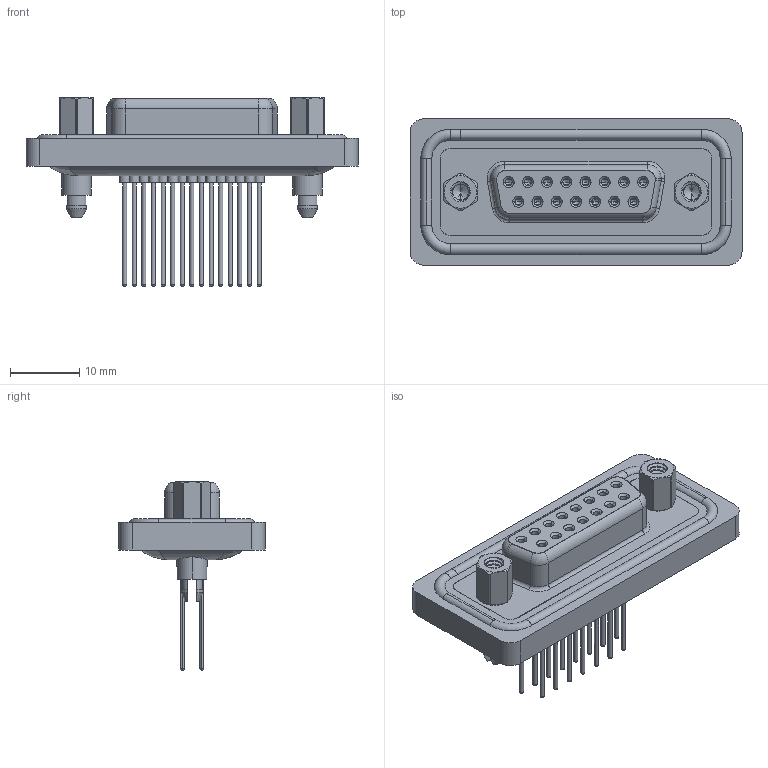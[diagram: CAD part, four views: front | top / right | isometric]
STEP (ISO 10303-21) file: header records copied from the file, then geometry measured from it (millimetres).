
FILE_DESCRIPTION (( 'STEP AP203' ), '1' );
FILE_NAME ('628-W15-321-013.STEP', '2020-09-11T23:25:36', ( '' ), ( '' ), 'SwSTEP 2.0', 'SolidWorks 2020', '' );
FILE_SCHEMA (( 'CONFIG_CONTROL_DESIGN' ));
Length unit declared in the file: millimetre
Products named in the file (8): 628W Housing_15 Contacts; 628W Waterproof Housing_15 Contacts BL; 628W Contact Row 1_21; 628W 4-40 Threaded Boardlock; 628W 4-40 Hex Standoff; 628-W15-321-013; 628W Contact Row 2_21; 628W Shell Front_15 Contacts
Assembly tree (22 placements, depth 2):
  628-W15-321-013
    628W Housing_15 Contacts
    628W Shell Front_15 Contacts
    628W Contact Row 1_21  x8
    628W Contact Row 2_21  x7
    628W 4-40 Threaded Boardlock  x2
    628W Waterproof Housing_15 Contacts BL
    628W 4-40 Hex Standoff  x2
Bounding box: 47.89 x 21.1 x 27.2 mm (x, y, z)
Volume: 5651.1 mm3; surface area: 9963.2 mm2
Topology: 23 solids, 23 shells, 1324 faces, 3196 edges, 1989 vertices
Faces by surface type: cylinder 563, plane 340, torus 260, cone 139, bspline 22
Entity records: 25350 total; most frequent: CARTESIAN_POINT 8378, DIRECTION 3481, ORIENTED_EDGE 3178, EDGE_CURVE 1589, AXIS2_PLACEMENT_3D 1441, VERTEX_POINT 1014, EDGE_LOOP 795, CIRCLE 772
